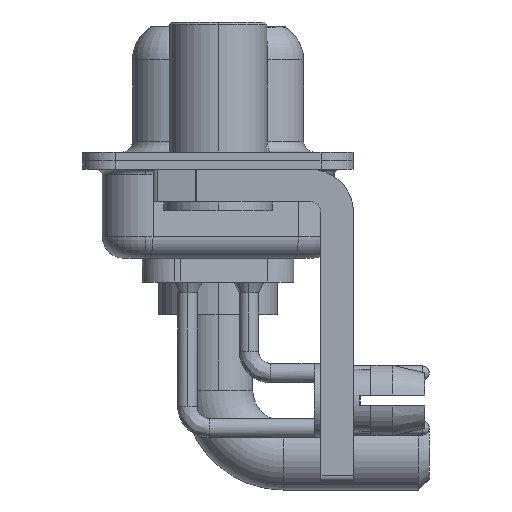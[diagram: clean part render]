
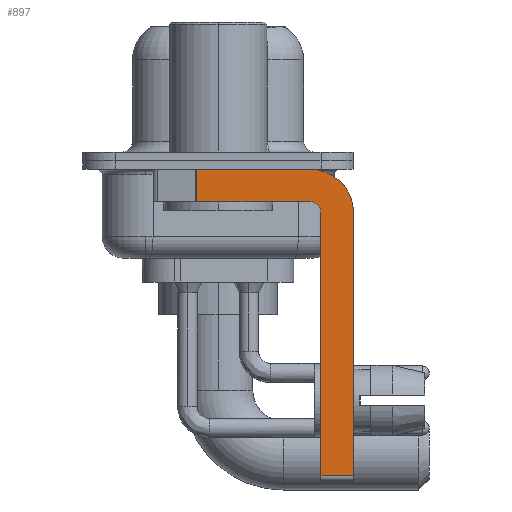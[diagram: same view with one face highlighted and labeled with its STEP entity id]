
A CAD part, left-side view. The second image highlights one B-rep face of the part: STEP entity #897.
In plain terms, the highlighted planar face has unit normal (-1, 0, 0).
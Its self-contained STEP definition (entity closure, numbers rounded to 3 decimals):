
#391 = DIRECTION ( 'NONE',  ( 0., 0., -1. ) ) ;
#810 = VECTOR ( 'NONE', #391, 1000. ) ;
#829 = DIRECTION ( 'NONE',  ( 0., -1., 0. ) ) ;
#897 = ADVANCED_FACE ( 'NONE', ( #5841 ), #16163, .F. ) ;
#898 = DIRECTION ( 'NONE',  ( 0., 0., 1. ) ) ;
#936 = CARTESIAN_POINT ( 'NONE',  ( -2.9, -4.25, -14.55 ) ) ;
#1511 = CARTESIAN_POINT ( 'NONE',  ( -2.9, -4.75, -2.4 ) ) ;
#1729 = VERTEX_POINT ( 'NONE', #2499 ) ;
#2056 = EDGE_CURVE ( 'NONE', #19736, #5551, #12010, .T. ) ;
#2456 = DIRECTION ( 'NONE',  ( 0., 1., 0. ) ) ;
#2499 = CARTESIAN_POINT ( 'NONE',  ( -2.9, -6.25, -14.55 ) ) ;
#2715 = CARTESIAN_POINT ( 'NONE',  ( -2.9, -4.25, -2.4 ) ) ;
#3163 = ORIENTED_EDGE ( 'NONE', *, *, #10281, .F. ) ;
#3225 = EDGE_CURVE ( 'NONE', #19162, #6417, #5832, .T. ) ;
#3544 = VECTOR ( 'NONE', #2456, 1000. ) ;
#3551 = CARTESIAN_POINT ( 'NONE',  ( -2.9, -6.25, -2.4 ) ) ;
#3899 = ORIENTED_EDGE ( 'NONE', *, *, #7347, .F. ) ;
#5179 = VERTEX_POINT ( 'NONE', #1511 ) ;
#5398 = DIRECTION ( 'NONE',  ( 0., -1., 0. ) ) ;
#5443 = CARTESIAN_POINT ( 'NONE',  ( -2.9, -6.25, -2.4 ) ) ;
#5551 = VERTEX_POINT ( 'NONE', #7455 ) ;
#5832 = LINE ( 'NONE', #16259, #3544 ) ;
#5841 = FACE_OUTER_BOUND ( 'NONE', #19117, .T. ) ;
#6062 = DIRECTION ( 'NONE',  ( 1., 0., 0. ) ) ;
#6417 = VERTEX_POINT ( 'NONE', #19264 ) ;
#6969 = DIRECTION ( 'NONE',  ( -1., 0., 0. ) ) ;
#7347 = EDGE_CURVE ( 'NONE', #5179, #19162, #21330, .T. ) ;
#7377 = LINE ( 'NONE', #3551, #810 ) ;
#7421 = CARTESIAN_POINT ( 'NONE',  ( -2.9, 0.978, -0.4 ) ) ;
#7455 = CARTESIAN_POINT ( 'NONE',  ( -2.9, -4.25, -0.4 ) ) ;
#8301 = DIRECTION ( 'NONE',  ( 0., 0., 1. ) ) ;
#8532 = CARTESIAN_POINT ( 'NONE',  ( -2.9, -4.75, -14.55 ) ) ;
#8871 = ORIENTED_EDGE ( 'NONE', *, *, #21993, .F. ) ;
#9540 = DIRECTION ( 'NONE',  ( 1., 0., 0. ) ) ;
#9886 = VECTOR ( 'NONE', #829, 1000. ) ;
#10281 = EDGE_CURVE ( 'NONE', #5551, #10708, #10971, .T. ) ;
#10708 = VERTEX_POINT ( 'NONE', #5443 ) ;
#10971 = CIRCLE ( 'NONE', #15625, 2. ) ;
#11022 = DIRECTION ( 'NONE',  ( 0., 0., -1. ) ) ;
#11277 = CARTESIAN_POINT ( 'NONE',  ( -2.9, 0.978, -1.9 ) ) ;
#11553 = EDGE_CURVE ( 'NONE', #15096, #5179, #16291, .T. ) ;
#11569 = ORIENTED_EDGE ( 'NONE', *, *, #3225, .F. ) ;
#12010 = LINE ( 'NONE', #13815, #15333 ) ;
#12358 = ORIENTED_EDGE ( 'NONE', *, *, #21788, .T. ) ;
#13080 = LINE ( 'NONE', #11277, #14446 ) ;
#13581 = CARTESIAN_POINT ( 'NONE',  ( -2.9, -4.25, -2.4 ) ) ;
#13815 = CARTESIAN_POINT ( 'NONE',  ( -2.9, 3., -0.4 ) ) ;
#14325 = EDGE_CURVE ( 'NONE', #15096, #1729, #18005, .T. ) ;
#14446 = VECTOR ( 'NONE', #14549, 1000. ) ;
#14549 = DIRECTION ( 'NONE',  ( 0., 0., -1. ) ) ;
#15096 = VERTEX_POINT ( 'NONE', #8532 ) ;
#15333 = VECTOR ( 'NONE', #5398, 1000. ) ;
#15625 = AXIS2_PLACEMENT_3D ( 'NONE', #2715, #9540, #11022 ) ;
#15669 = ORIENTED_EDGE ( 'NONE', *, *, #14325, .T. ) ;
#16072 = AXIS2_PLACEMENT_3D ( 'NONE', #21445, #6062, #18050 ) ;
#16163 = PLANE ( 'NONE',  #16072 ) ;
#16259 = CARTESIAN_POINT ( 'NONE',  ( -2.9, -4.25, -1.9 ) ) ;
#16291 = LINE ( 'NONE', #21584, #19187 ) ;
#17639 = ORIENTED_EDGE ( 'NONE', *, *, #2056, .F. ) ;
#18005 = LINE ( 'NONE', #936, #9886 ) ;
#18050 = DIRECTION ( 'NONE',  ( 0., 0., -1. ) ) ;
#18805 = AXIS2_PLACEMENT_3D ( 'NONE', #13581, #6969, #8301 ) ;
#19117 = EDGE_LOOP ( 'NONE', ( #17639, #12358, #11569, #3899, #20815, #15669, #8871, #3163 ) ) ;
#19162 = VERTEX_POINT ( 'NONE', #20558 ) ;
#19187 = VECTOR ( 'NONE', #898, 1000. ) ;
#19264 = CARTESIAN_POINT ( 'NONE',  ( -2.9, 0.978, -1.9 ) ) ;
#19736 = VERTEX_POINT ( 'NONE', #7421 ) ;
#20558 = CARTESIAN_POINT ( 'NONE',  ( -2.9, -4.25, -1.9 ) ) ;
#20815 = ORIENTED_EDGE ( 'NONE', *, *, #11553, .F. ) ;
#21330 = CIRCLE ( 'NONE', #18805, 0.5 ) ;
#21445 = CARTESIAN_POINT ( 'NONE',  ( -2.9, -4.25, -2.4 ) ) ;
#21584 = CARTESIAN_POINT ( 'NONE',  ( -2.9, -4.75, -14.8 ) ) ;
#21788 = EDGE_CURVE ( 'NONE', #19736, #6417, #13080, .T. ) ;
#21993 = EDGE_CURVE ( 'NONE', #10708, #1729, #7377, .T. ) ;
